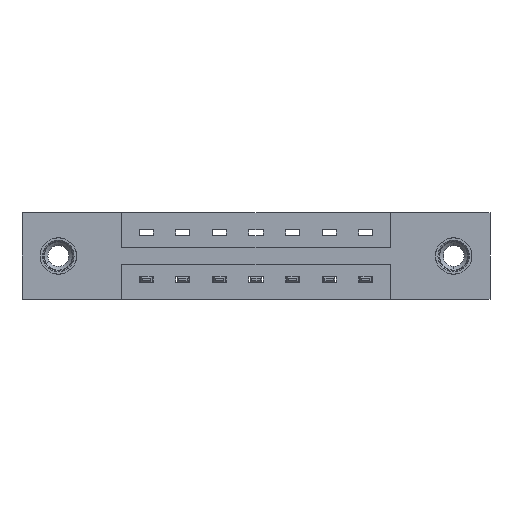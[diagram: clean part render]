
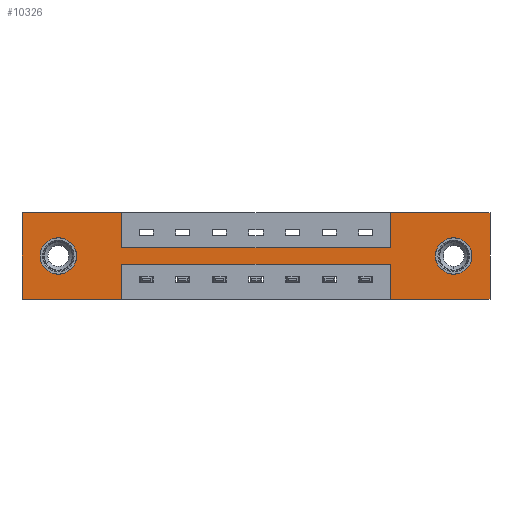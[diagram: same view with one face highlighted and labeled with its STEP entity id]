
A CAD part, front view. The second image highlights one B-rep face of the part: STEP entity #10326.
In plain terms, the highlighted planar face has unit normal (0, -1, 0).
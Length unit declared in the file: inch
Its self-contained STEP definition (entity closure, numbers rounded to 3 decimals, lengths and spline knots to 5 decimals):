
#36 = CIRCLE ( 'NONE', #8828, 0.078 ) ;
#140 = ORIENTED_EDGE ( 'NONE', *, *, #5518, .F. ) ;
#156 = DIRECTION ( 'NONE',  ( 0., 0., -1. ) ) ;
#186 = EDGE_LOOP ( 'NONE', ( #1166, #3827 ) ) ;
#363 = ORIENTED_EDGE ( 'NONE', *, *, #4164, .F. ) ;
#390 = ORIENTED_EDGE ( 'NONE', *, *, #6212, .F. ) ;
#418 = VERTEX_POINT ( 'NONE', #4861 ) ;
#453 = ORIENTED_EDGE ( 'NONE', *, *, #817, .F. ) ;
#464 = LINE ( 'NONE', #4411, #5233 ) ;
#543 = CARTESIAN_POINT ( 'NONE',  ( 0., 0., 0. ) ) ;
#553 = CARTESIAN_POINT ( 'NONE',  ( 0.425, 0., -0.15 ) ) ;
#590 = VERTEX_POINT ( 'NONE', #5624 ) ;
#686 = DIRECTION ( 'NONE',  ( 0., 0., -1. ) ) ;
#761 = VERTEX_POINT ( 'NONE', #3898 ) ;
#805 = VERTEX_POINT ( 'NONE', #1986 ) ;
#812 = CIRCLE ( 'NONE', #10600, 0.078 ) ;
#817 = EDGE_CURVE ( 'NONE', #5197, #4789, #8263, .T. ) ;
#838 = ORIENTED_EDGE ( 'NONE', *, *, #1145, .F. ) ;
#909 = EDGE_CURVE ( 'NONE', #805, #5197, #5356, .T. ) ;
#999 = EDGE_CURVE ( 'NONE', #6235, #4007, #2424, .T. ) ;
#1145 = EDGE_CURVE ( 'NONE', #761, #8175, #9630, .T. ) ;
#1166 = ORIENTED_EDGE ( 'NONE', *, *, #8496, .T. ) ;
#1169 = VECTOR ( 'NONE', #7746, 39.37008 ) ;
#1341 = LINE ( 'NONE', #10116, #9887 ) ;
#1364 = CARTESIAN_POINT ( 'NONE',  ( 0.425, 0., -0.37 ) ) ;
#1497 = ORIENTED_EDGE ( 'NONE', *, *, #9355, .F. ) ;
#1514 = LINE ( 'NONE', #4551, #10023 ) ;
#1553 = DIRECTION ( 'NONE',  ( 0., 0., -1. ) ) ;
#1573 = CARTESIAN_POINT ( 'NONE',  ( 1.573, 0., -0.37 ) ) ;
#1809 = VECTOR ( 'NONE', #8010, 39.37008 ) ;
#1853 = VERTEX_POINT ( 'NONE', #10329 ) ;
#1881 = DIRECTION ( 'NONE',  ( -1., 0., 0. ) ) ;
#1925 = CARTESIAN_POINT ( 'NONE',  ( 1.573, 0., -0.22 ) ) ;
#1986 = CARTESIAN_POINT ( 'NONE',  ( 0.425, 0., -0.22 ) ) ;
#2102 = LINE ( 'NONE', #7990, #1809 ) ;
#2157 = VECTOR ( 'NONE', #9825, 39.37008 ) ;
#2162 = CARTESIAN_POINT ( 'NONE',  ( 0., 0., -0.37 ) ) ;
#2424 = LINE ( 'NONE', #4693, #2157 ) ;
#2432 = CARTESIAN_POINT ( 'NONE',  ( 0.425, 0., 0. ) ) ;
#2488 = ORIENTED_EDGE ( 'NONE', *, *, #8884, .F. ) ;
#2678 = LINE ( 'NONE', #6975, #6965 ) ;
#2718 = EDGE_LOOP ( 'NONE', ( #7840, #4405, #7648, #9308, #2488, #1497, #363, #140, #390, #838, #4753, #453 ) ) ;
#2744 = VECTOR ( 'NONE', #4119, 39.37008 ) ;
#2824 = VECTOR ( 'NONE', #10468, 39.37008 ) ;
#2998 = FACE_BOUND ( 'NONE', #186, .T. ) ;
#3211 = DIRECTION ( 'NONE',  ( 1., 0., 0. ) ) ;
#3279 = EDGE_LOOP ( 'NONE', ( #10184, #3889 ) ) ;
#3695 = DIRECTION ( 'NONE',  ( 0., 0., -1. ) ) ;
#3709 = DIRECTION ( 'NONE',  ( -1., 0., 0. ) ) ;
#3827 = ORIENTED_EDGE ( 'NONE', *, *, #6127, .T. ) ;
#3889 = ORIENTED_EDGE ( 'NONE', *, *, #5762, .T. ) ;
#3898 = CARTESIAN_POINT ( 'NONE',  ( 0., 0., 0. ) ) ;
#3904 = VERTEX_POINT ( 'NONE', #10166 ) ;
#3954 = DIRECTION ( 'NONE',  ( 0., 1., 0. ) ) ;
#3986 = AXIS2_PLACEMENT_3D ( 'NONE', #10159, #5553, #156 ) ;
#3991 = CARTESIAN_POINT ( 'NONE',  ( 1.843, 0., -0.107 ) ) ;
#4007 = VERTEX_POINT ( 'NONE', #1925 ) ;
#4047 = VERTEX_POINT ( 'NONE', #4638 ) ;
#4079 = EDGE_CURVE ( 'NONE', #4007, #805, #2678, .T. ) ;
#4084 = CARTESIAN_POINT ( 'NONE',  ( 0.155, 0., -0.185 ) ) ;
#4119 = DIRECTION ( 'NONE',  ( 0., 0., 1. ) ) ;
#4164 = EDGE_CURVE ( 'NONE', #6140, #3904, #2102, .T. ) ;
#4209 = CARTESIAN_POINT ( 'NONE',  ( 0., 0., -0.37 ) ) ;
#4366 = CARTESIAN_POINT ( 'NONE',  ( 0.425, 0., 0. ) ) ;
#4405 = ORIENTED_EDGE ( 'NONE', *, *, #4079, .F. ) ;
#4411 = CARTESIAN_POINT ( 'NONE',  ( 0., 0., 0. ) ) ;
#4447 = LINE ( 'NONE', #2432, #10494 ) ;
#4551 = CARTESIAN_POINT ( 'NONE',  ( 0., 0., -0.37 ) ) ;
#4638 = CARTESIAN_POINT ( 'NONE',  ( 0.425, 0., -0.15 ) ) ;
#4693 = CARTESIAN_POINT ( 'NONE',  ( 1.573, 0., -0.37 ) ) ;
#4753 = ORIENTED_EDGE ( 'NONE', *, *, #9170, .F. ) ;
#4789 = VERTEX_POINT ( 'NONE', #10478 ) ;
#4848 = AXIS2_PLACEMENT_3D ( 'NONE', #10052, #5410, #686 ) ;
#4861 = CARTESIAN_POINT ( 'NONE',  ( 1.998, 0., -0.37 ) ) ;
#4961 = DIRECTION ( 'NONE',  ( 0., 0., 1. ) ) ;
#5147 = EDGE_CURVE ( 'NONE', #418, #6235, #1514, .T. ) ;
#5169 = LINE ( 'NONE', #553, #2824 ) ;
#5197 = VERTEX_POINT ( 'NONE', #9417 ) ;
#5233 = VECTOR ( 'NONE', #9976, 39.37008 ) ;
#5356 = LINE ( 'NONE', #1364, #1169 ) ;
#5405 = VERTEX_POINT ( 'NONE', #3991 ) ;
#5410 = DIRECTION ( 'NONE',  ( 0., 1., 0. ) ) ;
#5518 = EDGE_CURVE ( 'NONE', #4047, #6140, #5169, .T. ) ;
#5553 = DIRECTION ( 'NONE',  ( 0., 1., 0. ) ) ;
#5624 = CARTESIAN_POINT ( 'NONE',  ( 1.998, 0., 0. ) ) ;
#5648 = CARTESIAN_POINT ( 'NONE',  ( 0.155, 0., -0.107 ) ) ;
#5762 = EDGE_CURVE ( 'NONE', #1853, #5405, #9240, .T. ) ;
#5987 = PLANE ( 'NONE',  #10484 ) ;
#6127 = EDGE_CURVE ( 'NONE', #7565, #8982, #812, .T. ) ;
#6140 = VERTEX_POINT ( 'NONE', #6654 ) ;
#6212 = EDGE_CURVE ( 'NONE', #8175, #4047, #4447, .T. ) ;
#6235 = VERTEX_POINT ( 'NONE', #1573 ) ;
#6654 = CARTESIAN_POINT ( 'NONE',  ( 1.573, 0., -0.15 ) ) ;
#6755 = DIRECTION ( 'NONE',  ( 0., 0., -1. ) ) ;
#6769 = DIRECTION ( 'NONE',  ( 0., -1., 0. ) ) ;
#6965 = VECTOR ( 'NONE', #8036, 39.37008 ) ;
#6975 = CARTESIAN_POINT ( 'NONE',  ( 0.425, 0., -0.22 ) ) ;
#7041 = EDGE_CURVE ( 'NONE', #5405, #1853, #10251, .T. ) ;
#7498 = FACE_BOUND ( 'NONE', #3279, .T. ) ;
#7526 = LINE ( 'NONE', #543, #2744 ) ;
#7565 = VERTEX_POINT ( 'NONE', #8512 ) ;
#7627 = VECTOR ( 'NONE', #3211, 39.37008 ) ;
#7648 = ORIENTED_EDGE ( 'NONE', *, *, #999, .F. ) ;
#7746 = DIRECTION ( 'NONE',  ( 0., 0., -1. ) ) ;
#7840 = ORIENTED_EDGE ( 'NONE', *, *, #909, .F. ) ;
#7990 = CARTESIAN_POINT ( 'NONE',  ( 1.573, 0., 0. ) ) ;
#8006 = VECTOR ( 'NONE', #1881, 39.37008 ) ;
#8010 = DIRECTION ( 'NONE',  ( 0., 0., 1. ) ) ;
#8036 = DIRECTION ( 'NONE',  ( -1., 0., 0. ) ) ;
#8175 = VERTEX_POINT ( 'NONE', #4366 ) ;
#8263 = LINE ( 'NONE', #2162, #8006 ) ;
#8496 = EDGE_CURVE ( 'NONE', #8982, #7565, #36, .T. ) ;
#8512 = CARTESIAN_POINT ( 'NONE',  ( 0.155, 0., -0.263 ) ) ;
#8828 = AXIS2_PLACEMENT_3D ( 'NONE', #8848, #3954, #9573 ) ;
#8848 = CARTESIAN_POINT ( 'NONE',  ( 0.155, 0., -0.185 ) ) ;
#8884 = EDGE_CURVE ( 'NONE', #590, #418, #1341, .T. ) ;
#8982 = VERTEX_POINT ( 'NONE', #5648 ) ;
#9059 = CARTESIAN_POINT ( 'NONE',  ( 0., 0., 0. ) ) ;
#9170 = EDGE_CURVE ( 'NONE', #4789, #761, #7526, .T. ) ;
#9240 = CIRCLE ( 'NONE', #4848, 0.078 ) ;
#9269 = FACE_OUTER_BOUND ( 'NONE', #2718, .T. ) ;
#9308 = ORIENTED_EDGE ( 'NONE', *, *, #5147, .F. ) ;
#9355 = EDGE_CURVE ( 'NONE', #3904, #590, #464, .T. ) ;
#9417 = CARTESIAN_POINT ( 'NONE',  ( 0.425, 0., -0.37 ) ) ;
#9573 = DIRECTION ( 'NONE',  ( 0., 0., 1. ) ) ;
#9630 = LINE ( 'NONE', #9059, #7627 ) ;
#9693 = DIRECTION ( 'NONE',  ( 0., 1., 0. ) ) ;
#9825 = DIRECTION ( 'NONE',  ( 0., 0., 1. ) ) ;
#9887 = VECTOR ( 'NONE', #3695, 39.37008 ) ;
#9976 = DIRECTION ( 'NONE',  ( 1., 0., 0. ) ) ;
#10023 = VECTOR ( 'NONE', #3709, 39.37008 ) ;
#10052 = CARTESIAN_POINT ( 'NONE',  ( 1.843, 0., -0.185 ) ) ;
#10116 = CARTESIAN_POINT ( 'NONE',  ( 1.998, 0., 0. ) ) ;
#10159 = CARTESIAN_POINT ( 'NONE',  ( 1.843, 0., -0.185 ) ) ;
#10166 = CARTESIAN_POINT ( 'NONE',  ( 1.573, 0., 0. ) ) ;
#10184 = ORIENTED_EDGE ( 'NONE', *, *, #7041, .T. ) ;
#10251 = CIRCLE ( 'NONE', #3986, 0.078 ) ;
#10326 = ADVANCED_FACE ( 'NONE', ( #7498, #2998, #9269 ), #5987, .T. ) ;
#10329 = CARTESIAN_POINT ( 'NONE',  ( 1.843, 0., -0.263 ) ) ;
#10468 = DIRECTION ( 'NONE',  ( 1., 0., 0. ) ) ;
#10478 = CARTESIAN_POINT ( 'NONE',  ( 0., 0., -0.37 ) ) ;
#10484 = AXIS2_PLACEMENT_3D ( 'NONE', #4209, #6769, #1553 ) ;
#10494 = VECTOR ( 'NONE', #6755, 39.37008 ) ;
#10600 = AXIS2_PLACEMENT_3D ( 'NONE', #4084, #9693, #4961 ) ;
